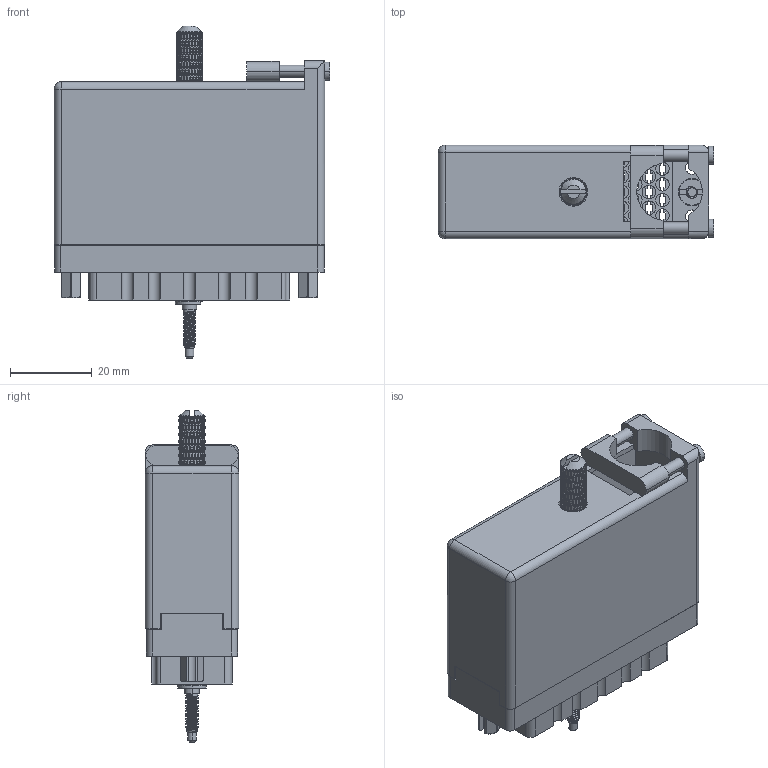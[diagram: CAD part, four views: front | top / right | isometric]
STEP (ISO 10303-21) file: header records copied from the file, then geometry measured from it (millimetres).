
FILE_DESCRIPTION (( 'STEP AP203' ), '1' );
FILE_NAME ('516-056-000-261.STEP', '2020-03-05T19:47:31', ( '' ), ( '' ), 'SwSTEP 2.0', 'SolidWorks 2016', '' );
FILE_SCHEMA (( 'CONFIG_CONTROL_DESIGN' ));
Products named in the file (11): 516-251-035-100; 516-230-001_Metal - 056 Top Entry; 516-221-038-102_057; Actuating Screw Assy 038-056; 516-221-038-102_056; 516-250-038-111; 516-056-000-261; 516-252-021-102_056; 516-253-138-107; 516-253-035-100; 516 Part Receptacle_056
Assembly tree (12 placements, depth 3):
  516-056-000-261
    516 Part Receptacle_056
    516-230-001_Metal - 056 Top Entry
    516-252-021-102_056  x2
    516-221-038-102_056
    Actuating Screw Assy 038-056
      516-251-035-100
      516-253-035-100  x2
      516-253-138-107
      516-250-038-111
    516-221-038-102_057
Bounding box: 67.31 x 22.83 x 81.03 mm (x, y, z)
Volume: 27128.1 mm3; surface area: 39466 mm2
Topology: 11 solids, 11 shells, 2896 faces, 7370 edges, 4510 vertices
Faces by surface type: plane 1049, bspline 1034, cylinder 759, cone 52, sphere 2
Entity records: 120310 total; most frequent: CARTESIAN_POINT 61334, ORIENTED_EDGE 14524, DIRECTION 9425, EDGE_CURVE 7262, VERTEX_POINT 4442, AXIS2_PLACEMENT_3D 3159, VECTOR 3107, LINE 3107
